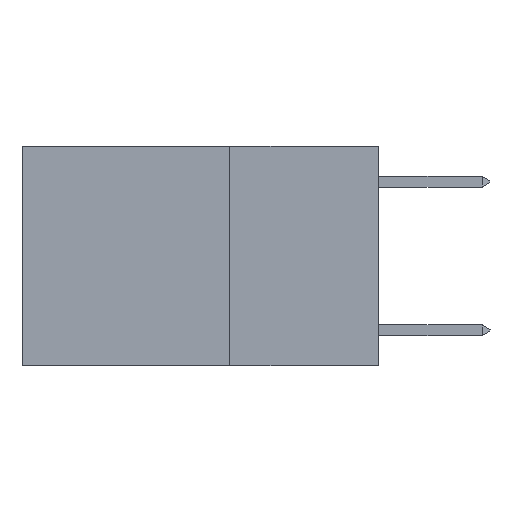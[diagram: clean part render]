
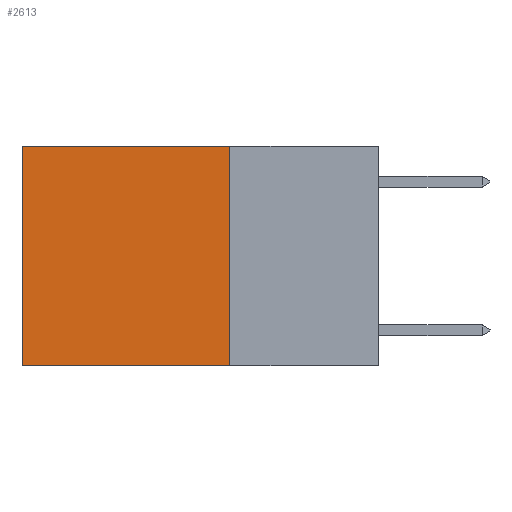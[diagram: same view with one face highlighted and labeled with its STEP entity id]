
A CAD part, left-side view. The second image highlights one B-rep face of the part: STEP entity #2613.
In plain terms, the highlighted planar face has unit normal (-1, 0, 0).
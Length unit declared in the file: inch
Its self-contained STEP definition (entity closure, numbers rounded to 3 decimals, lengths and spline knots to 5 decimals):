
#228 = VECTOR ( 'NONE', #14915, 39.37008 ) ;
#249 = ORIENTED_EDGE ( 'NONE', *, *, #16389, .F. ) ;
#752 = VECTOR ( 'NONE', #14511, 39.37008 ) ;
#2466 = CARTESIAN_POINT ( 'NONE',  ( 0.2625, 0.25, 0. ) ) ;
#2511 = CARTESIAN_POINT ( 'NONE',  ( 0.2625, 0.25, -0.37 ) ) ;
#2613 = ADVANCED_FACE ( 'NONE', ( #8643 ), #15691, .F. ) ;
#3574 = EDGE_CURVE ( 'NONE', #11881, #18312, #16033, .T. ) ;
#3646 = EDGE_LOOP ( 'NONE', ( #13622, #249, #15900, #18469 ) ) ;
#3979 = LINE ( 'NONE', #14757, #15856 ) ;
#5727 = LINE ( 'NONE', #8538, #752 ) ;
#5947 = VERTEX_POINT ( 'NONE', #2466 ) ;
#6233 = CARTESIAN_POINT ( 'NONE',  ( 0.2625, 0.6, -0.37 ) ) ;
#6804 = DIRECTION ( 'NONE',  ( 1., 0., 0. ) ) ;
#7499 = CARTESIAN_POINT ( 'NONE',  ( 0.2625, 0.25, -0.37 ) ) ;
#8538 = CARTESIAN_POINT ( 'NONE',  ( 0.2625, 0.25, 0. ) ) ;
#8643 = FACE_OUTER_BOUND ( 'NONE', #3646, .T. ) ;
#8968 = DIRECTION ( 'NONE',  ( 0., 0., -1. ) ) ;
#9259 = EDGE_CURVE ( 'NONE', #5947, #15485, #3979, .T. ) ;
#11881 = VERTEX_POINT ( 'NONE', #14702 ) ;
#12143 = VECTOR ( 'NONE', #8968, 39.37008 ) ;
#13606 = LINE ( 'NONE', #7499, #228 ) ;
#13622 = ORIENTED_EDGE ( 'NONE', *, *, #3574, .T. ) ;
#14511 = DIRECTION ( 'NONE',  ( 0., 1., 0. ) ) ;
#14702 = CARTESIAN_POINT ( 'NONE',  ( 0.2625, 0.6, 0. ) ) ;
#14757 = CARTESIAN_POINT ( 'NONE',  ( 0.2625, 0.25, 0. ) ) ;
#14915 = DIRECTION ( 'NONE',  ( 0., 1., 0. ) ) ;
#14982 = EDGE_CURVE ( 'NONE', #5947, #11881, #5727, .T. ) ;
#15437 = AXIS2_PLACEMENT_3D ( 'NONE', #17098, #6804, #17166 ) ;
#15485 = VERTEX_POINT ( 'NONE', #2511 ) ;
#15691 = PLANE ( 'NONE',  #15437 ) ;
#15856 = VECTOR ( 'NONE', #16252, 39.37008 ) ;
#15900 = ORIENTED_EDGE ( 'NONE', *, *, #9259, .F. ) ;
#16033 = LINE ( 'NONE', #19220, #12143 ) ;
#16252 = DIRECTION ( 'NONE',  ( 0., 0., -1. ) ) ;
#16389 = EDGE_CURVE ( 'NONE', #15485, #18312, #13606, .T. ) ;
#17098 = CARTESIAN_POINT ( 'NONE',  ( 0.2625, 0.25, 0. ) ) ;
#17166 = DIRECTION ( 'NONE',  ( 0., 0., -1. ) ) ;
#18312 = VERTEX_POINT ( 'NONE', #6233 ) ;
#18469 = ORIENTED_EDGE ( 'NONE', *, *, #14982, .T. ) ;
#19220 = CARTESIAN_POINT ( 'NONE',  ( 0.2625, 0.6, 0. ) ) ;
